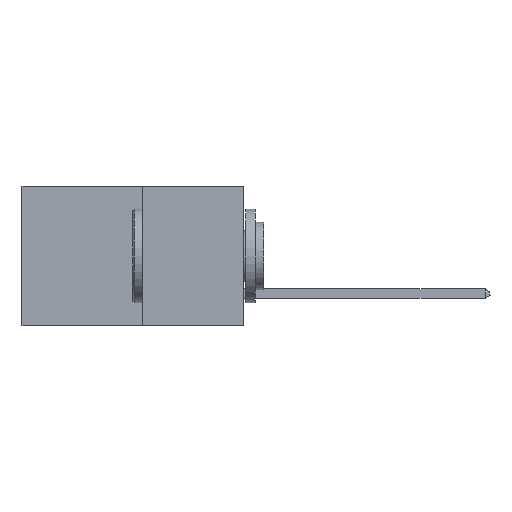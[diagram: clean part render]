
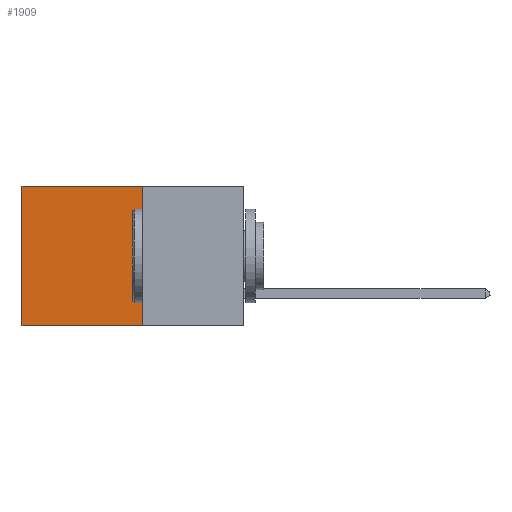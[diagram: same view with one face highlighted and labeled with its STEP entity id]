
A CAD part, left-side view. The second image highlights one B-rep face of the part: STEP entity #1909.
In plain terms, the highlighted planar face has unit normal (-1, 0, 0).
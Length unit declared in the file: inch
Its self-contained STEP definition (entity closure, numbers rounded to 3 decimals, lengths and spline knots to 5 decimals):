
#488 = LINE ( 'NONE', #4513, #5584 ) ;
#787 = VECTOR ( 'NONE', #9833, 39.37008 ) ;
#1485 = VERTEX_POINT ( 'NONE', #6691 ) ;
#1909 = ADVANCED_FACE ( 'NONE', ( #8304 ), #2025, .F. ) ;
#2025 = PLANE ( 'NONE',  #10854 ) ;
#2992 = CARTESIAN_POINT ( 'NONE',  ( 0.277, 0.27, -0.37 ) ) ;
#3484 = CARTESIAN_POINT ( 'NONE',  ( 0.277, 0.27, -0.37 ) ) ;
#3556 = DIRECTION ( 'NONE',  ( 1., 0., 0. ) ) ;
#3584 = VECTOR ( 'NONE', #6827, 39.37008 ) ;
#4106 = CARTESIAN_POINT ( 'NONE',  ( 0.277, 0.59, 0. ) ) ;
#4496 = DIRECTION ( 'NONE',  ( 0., 0., -1. ) ) ;
#4513 = CARTESIAN_POINT ( 'NONE',  ( 0.277, 0.59, -0.37 ) ) ;
#4661 = LINE ( 'NONE', #9044, #11745 ) ;
#4961 = CARTESIAN_POINT ( 'NONE',  ( 0.277, 0.27, -0.37 ) ) ;
#5331 = EDGE_CURVE ( 'NONE', #7150, #7190, #8873, .T. ) ;
#5584 = VECTOR ( 'NONE', #4496, 39.37008 ) ;
#5679 = DIRECTION ( 'NONE',  ( 0., 0., -1. ) ) ;
#6015 = CARTESIAN_POINT ( 'NONE',  ( 0.277, 0.27, 0. ) ) ;
#6194 = LINE ( 'NONE', #4961, #787 ) ;
#6248 = EDGE_CURVE ( 'NONE', #7190, #1485, #488, .T. ) ;
#6544 = ORIENTED_EDGE ( 'NONE', *, *, #6248, .T. ) ;
#6691 = CARTESIAN_POINT ( 'NONE',  ( 0.277, 0.59, -0.37 ) ) ;
#6827 = DIRECTION ( 'NONE',  ( 0., 1., 0. ) ) ;
#6895 = VERTEX_POINT ( 'NONE', #2992 ) ;
#6908 = CARTESIAN_POINT ( 'NONE',  ( 0.277, 0.27, 0. ) ) ;
#7150 = VERTEX_POINT ( 'NONE', #6015 ) ;
#7190 = VERTEX_POINT ( 'NONE', #4106 ) ;
#7753 = EDGE_CURVE ( 'NONE', #7150, #6895, #6194, .T. ) ;
#8304 = FACE_OUTER_BOUND ( 'NONE', #12235, .T. ) ;
#8728 = ORIENTED_EDGE ( 'NONE', *, *, #7753, .F. ) ;
#8873 = LINE ( 'NONE', #6908, #3584 ) ;
#9044 = CARTESIAN_POINT ( 'NONE',  ( 0.277, 0.27, -0.37 ) ) ;
#9734 = ORIENTED_EDGE ( 'NONE', *, *, #12349, .F. ) ;
#9833 = DIRECTION ( 'NONE',  ( 0., 0., -1. ) ) ;
#10854 = AXIS2_PLACEMENT_3D ( 'NONE', #3484, #3556, #5679 ) ;
#11200 = ORIENTED_EDGE ( 'NONE', *, *, #5331, .T. ) ;
#11745 = VECTOR ( 'NONE', #11837, 39.37008 ) ;
#11837 = DIRECTION ( 'NONE',  ( 0., 1., 0. ) ) ;
#12235 = EDGE_LOOP ( 'NONE', ( #6544, #9734, #8728, #11200 ) ) ;
#12349 = EDGE_CURVE ( 'NONE', #6895, #1485, #4661, .T. ) ;
